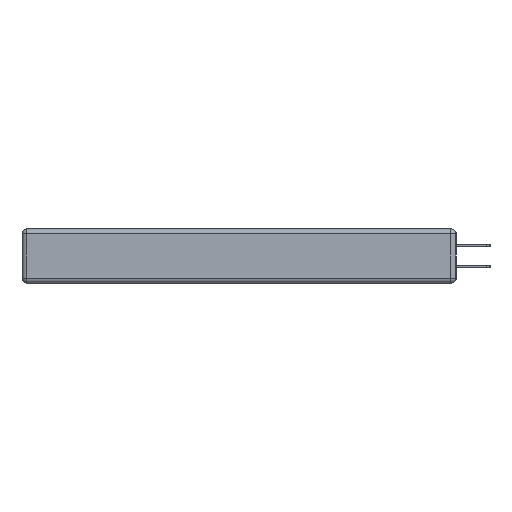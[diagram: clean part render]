
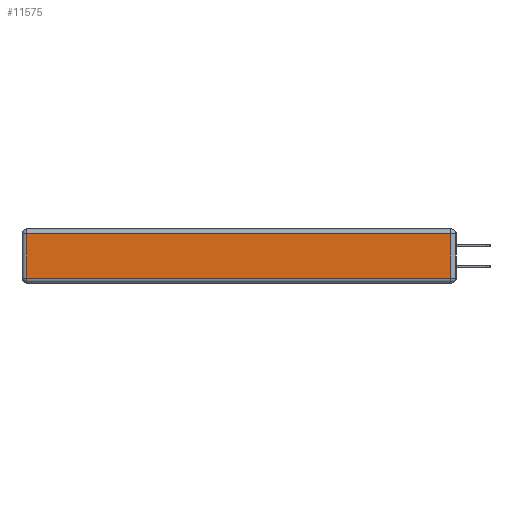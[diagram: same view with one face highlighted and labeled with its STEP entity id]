
A CAD part, left-side view. The second image highlights one B-rep face of the part: STEP entity #11575.
In plain terms, the highlighted planar face has unit normal (-1, 0, 0).
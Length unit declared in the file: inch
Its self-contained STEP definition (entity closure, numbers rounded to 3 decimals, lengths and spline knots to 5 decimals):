
#112 = ORIENTED_EDGE ( 'NONE', *, *, #550, .T. ) ;
#454 = ORIENTED_EDGE ( 'NONE', *, *, #19174, .T. ) ;
#550 = EDGE_CURVE ( 'NONE', #10253, #3750, #3167, .T. ) ;
#1690 = EDGE_CURVE ( 'NONE', #13104, #10253, #13241, .T. ) ;
#3167 = LINE ( 'NONE', #16439, #6464 ) ;
#3750 = VERTEX_POINT ( 'NONE', #10818 ) ;
#4116 = DIRECTION ( 'NONE',  ( 0., 0., -1. ) ) ;
#4201 = DIRECTION ( 'NONE',  ( -1., 0., 0. ) ) ;
#4492 = CARTESIAN_POINT ( 'NONE',  ( 0., 0., -0.313 ) ) ;
#6464 = VECTOR ( 'NONE', #7007, 39.37008 ) ;
#7007 = DIRECTION ( 'NONE',  ( 0., 1., 0. ) ) ;
#7154 = VERTEX_POINT ( 'NONE', #17699 ) ;
#7282 = VECTOR ( 'NONE', #16244, 39.37008 ) ;
#7797 = LINE ( 'NONE', #17690, #16687 ) ;
#8718 = LINE ( 'NONE', #4492, #7282 ) ;
#9556 = CARTESIAN_POINT ( 'NONE',  ( 0., 0.03, -0.03 ) ) ;
#10253 = VERTEX_POINT ( 'NONE', #9556 ) ;
#10350 = FACE_OUTER_BOUND ( 'NONE', #17661, .T. ) ;
#10403 = CARTESIAN_POINT ( 'NONE',  ( 0., 0.03, -0.313 ) ) ;
#10818 = CARTESIAN_POINT ( 'NONE',  ( 0., 2.72, -0.03 ) ) ;
#11575 = ADVANCED_FACE ( 'NONE', ( #10350 ), #17651, .T. ) ;
#11870 = CARTESIAN_POINT ( 'NONE',  ( 0., 0.03, -0.343 ) ) ;
#12275 = ORIENTED_EDGE ( 'NONE', *, *, #14811, .T. ) ;
#13104 = VERTEX_POINT ( 'NONE', #10403 ) ;
#13222 = CARTESIAN_POINT ( 'NONE',  ( 0., 0., -0.343 ) ) ;
#13241 = LINE ( 'NONE', #11870, #15521 ) ;
#14693 = DIRECTION ( 'NONE',  ( 0., 0., 1. ) ) ;
#14811 = EDGE_CURVE ( 'NONE', #7154, #13104, #8718, .T. ) ;
#15521 = VECTOR ( 'NONE', #16330, 39.37008 ) ;
#16244 = DIRECTION ( 'NONE',  ( 0., -1., 0. ) ) ;
#16330 = DIRECTION ( 'NONE',  ( 0., 0., 1. ) ) ;
#16439 = CARTESIAN_POINT ( 'NONE',  ( 0., 2.75, -0.03 ) ) ;
#16687 = VECTOR ( 'NONE', #4116, 39.37008 ) ;
#17363 = ORIENTED_EDGE ( 'NONE', *, *, #1690, .T. ) ;
#17651 = PLANE ( 'NONE',  #18165 ) ;
#17661 = EDGE_LOOP ( 'NONE', ( #12275, #17363, #112, #454 ) ) ;
#17690 = CARTESIAN_POINT ( 'NONE',  ( 0., 2.72, -0.343 ) ) ;
#17699 = CARTESIAN_POINT ( 'NONE',  ( 0., 2.72, -0.313 ) ) ;
#18165 = AXIS2_PLACEMENT_3D ( 'NONE', #13222, #4201, #14693 ) ;
#19174 = EDGE_CURVE ( 'NONE', #3750, #7154, #7797, .T. ) ;
